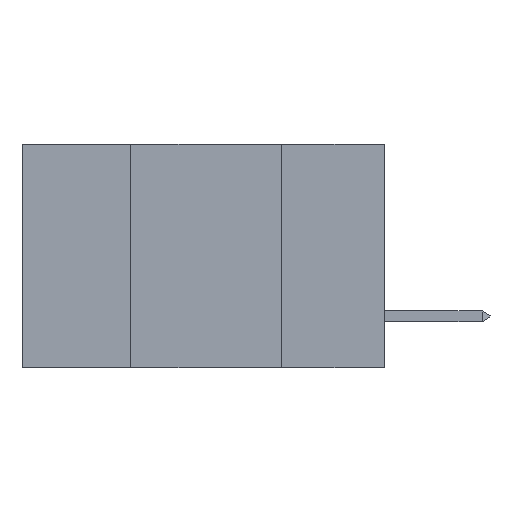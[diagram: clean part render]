
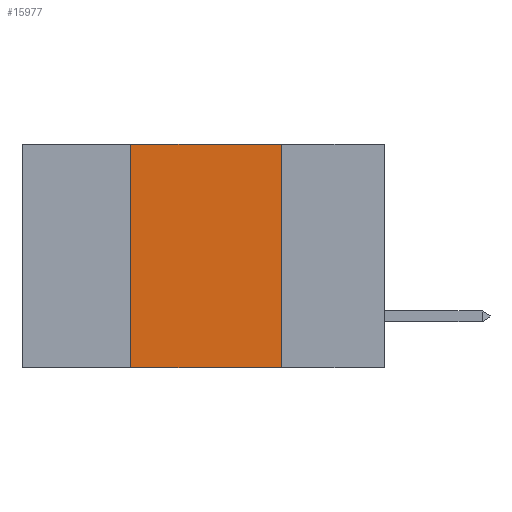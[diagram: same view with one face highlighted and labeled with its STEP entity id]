
A CAD part, left-side view. The second image highlights one B-rep face of the part: STEP entity #15977.
In plain terms, the highlighted planar face has unit normal (-1, 0, 0).
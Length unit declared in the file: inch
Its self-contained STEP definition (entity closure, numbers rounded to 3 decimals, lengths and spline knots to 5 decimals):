
#2205 = CARTESIAN_POINT ( 'NONE',  ( 0., 0.17, -0.37 ) ) ;
#2788 = EDGE_CURVE ( 'NONE', #31242, #16609, #5668, .T. ) ;
#5004 = ORIENTED_EDGE ( 'NONE', *, *, #2788, .T. ) ;
#5120 = EDGE_CURVE ( 'NONE', #31242, #18073, #18444, .T. ) ;
#5668 = LINE ( 'NONE', #27628, #19395 ) ;
#6589 = CARTESIAN_POINT ( 'NONE',  ( 0., 0.42, -0.37 ) ) ;
#7914 = VECTOR ( 'NONE', #19324, 39.37008 ) ;
#8289 = CARTESIAN_POINT ( 'NONE',  ( 0., 0.17, 0. ) ) ;
#8351 = CARTESIAN_POINT ( 'NONE',  ( 0., 0.6, 0. ) ) ;
#9228 = LINE ( 'NONE', #21726, #7914 ) ;
#9811 = ORIENTED_EDGE ( 'NONE', *, *, #24122, .F. ) ;
#10615 = VECTOR ( 'NONE', #20153, 39.37008 ) ;
#10925 = DIRECTION ( 'NONE',  ( 0., -1., 0. ) ) ;
#12529 = DIRECTION ( 'NONE',  ( 1., 0., 0. ) ) ;
#15447 = DIRECTION ( 'NONE',  ( 0., -1., 0. ) ) ;
#15977 = ADVANCED_FACE ( 'NONE', ( #20543 ), #30305, .F. ) ;
#16045 = LINE ( 'NONE', #18139, #24395 ) ;
#16609 = VERTEX_POINT ( 'NONE', #2205 ) ;
#18073 = VERTEX_POINT ( 'NONE', #30554 ) ;
#18139 = CARTESIAN_POINT ( 'NONE',  ( 0., 0.6, 0. ) ) ;
#18401 = EDGE_LOOP ( 'NONE', ( #9811, #28554, #22102, #5004 ) ) ;
#18444 = LINE ( 'NONE', #24643, #10615 ) ;
#19324 = DIRECTION ( 'NONE',  ( 0., 0., -1. ) ) ;
#19395 = VECTOR ( 'NONE', #15447, 39.37008 ) ;
#20153 = DIRECTION ( 'NONE',  ( 0., 0., 1. ) ) ;
#20543 = FACE_OUTER_BOUND ( 'NONE', #18401, .T. ) ;
#21726 = CARTESIAN_POINT ( 'NONE',  ( 0., 0.17, 0. ) ) ;
#22102 = ORIENTED_EDGE ( 'NONE', *, *, #5120, .F. ) ;
#22178 = VERTEX_POINT ( 'NONE', #8289 ) ;
#24122 = EDGE_CURVE ( 'NONE', #22178, #16609, #9228, .T. ) ;
#24395 = VECTOR ( 'NONE', #10925, 39.37008 ) ;
#24643 = CARTESIAN_POINT ( 'NONE',  ( 0., 0.42, 0. ) ) ;
#26129 = EDGE_CURVE ( 'NONE', #18073, #22178, #16045, .T. ) ;
#27280 = DIRECTION ( 'NONE',  ( 0., 0., -1. ) ) ;
#27628 = CARTESIAN_POINT ( 'NONE',  ( 0., 0.6, -0.37 ) ) ;
#28369 = AXIS2_PLACEMENT_3D ( 'NONE', #8351, #12529, #27280 ) ;
#28554 = ORIENTED_EDGE ( 'NONE', *, *, #26129, .F. ) ;
#30305 = PLANE ( 'NONE',  #28369 ) ;
#30554 = CARTESIAN_POINT ( 'NONE',  ( 0., 0.42, 0. ) ) ;
#31242 = VERTEX_POINT ( 'NONE', #6589 ) ;
